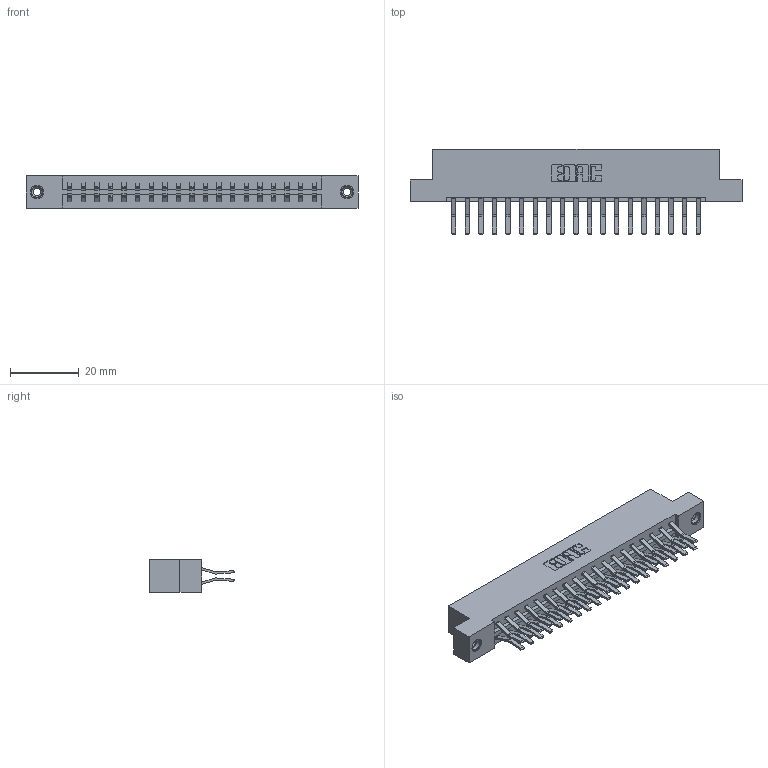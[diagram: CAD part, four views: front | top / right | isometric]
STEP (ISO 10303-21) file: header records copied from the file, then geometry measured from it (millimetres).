
FILE_DESCRIPTION (( 'STEP AP203' ), '1' );
FILE_NAME ('333-038-560-208.STEP', '2018-08-03T12:19:13', ( '' ), ( '' ), 'SwSTEP 2.0', 'SolidWorks 2016', '' );
FILE_SCHEMA (( 'CONFIG_CONTROL_DESIGN' ));
Length unit declared in the file: inch
Products named in the file (4): 345-292-001_560 Tail; 345-250-001_345-250-003-102; 333-038-560-208; 333 Part_Flush - .156 Dia - TI
Assembly tree (41 placements, depth 2):
  333-038-560-208
    333 Part_Flush - .156 Dia - TI
    345-292-001_560 Tail  x38
    345-250-001_345-250-003-102  x2
Bounding box: 96.82 x 24.78 x 9.4 mm (x, y, z)
Volume: 9912.7 mm3; surface area: 12204.4 mm2
Topology: 41 solids, 41 shells, 2226 faces, 6565 edges, 4318 vertices
Faces by surface type: plane 1470, cylinder 740, cone 12, torus 4
Entity records: 16472 total; most frequent: CARTESIAN_POINT 2741, ORIENTED_EDGE 2670, DIRECTION 2417, EDGE_CURVE 1335, LINE 1183, VECTOR 1183, VERTEX_POINT 884, AXIS2_PLACEMENT_3D 617
